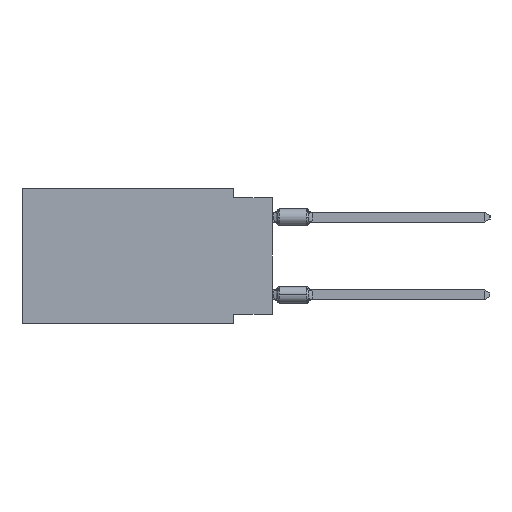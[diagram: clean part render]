
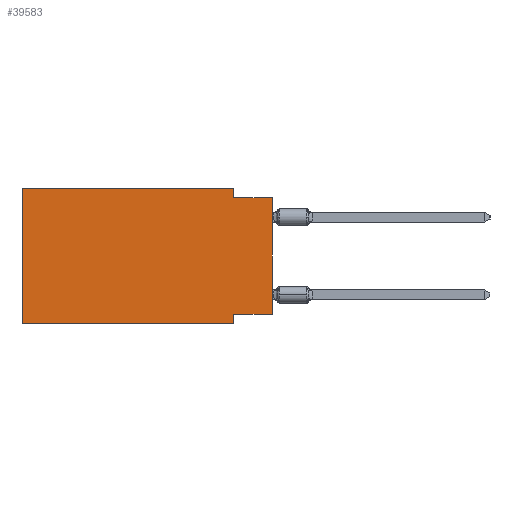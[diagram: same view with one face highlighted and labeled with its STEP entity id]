
A CAD part, left-side view. The second image highlights one B-rep face of the part: STEP entity #39583.
In plain terms, the highlighted planar face has unit normal (-1, 0, 0).
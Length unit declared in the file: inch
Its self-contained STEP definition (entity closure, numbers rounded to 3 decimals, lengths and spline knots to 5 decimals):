
#415 = CARTESIAN_POINT ( 'NONE',  ( 0., 0.1, -0.35 ) ) ;
#735 = DIRECTION ( 'NONE',  ( 0., 0., 1. ) ) ;
#1267 = FACE_OUTER_BOUND ( 'NONE', #35746, .T. ) ;
#1519 = VECTOR ( 'NONE', #735, 39.37008 ) ;
#1534 = EDGE_CURVE ( 'NONE', #35348, #14423, #10253, .T. ) ;
#1948 = EDGE_CURVE ( 'NONE', #33813, #29444, #14636, .T. ) ;
#2580 = DIRECTION ( 'NONE',  ( 0., -1., 0. ) ) ;
#2757 = CARTESIAN_POINT ( 'NONE',  ( 0., 0.1, -0.025 ) ) ;
#4021 = CARTESIAN_POINT ( 'NONE',  ( 0., 0., 0. ) ) ;
#4475 = LINE ( 'NONE', #37735, #1519 ) ;
#4509 = ORIENTED_EDGE ( 'NONE', *, *, #49030, .F. ) ;
#6438 = CARTESIAN_POINT ( 'NONE',  ( 0., 0.645, 0. ) ) ;
#8901 = VECTOR ( 'NONE', #40226, 39.37008 ) ;
#8943 = PLANE ( 'NONE',  #25062 ) ;
#10253 = LINE ( 'NONE', #26356, #43777 ) ;
#10476 = VERTEX_POINT ( 'NONE', #6438 ) ;
#10911 = ORIENTED_EDGE ( 'NONE', *, *, #32629, .F. ) ;
#11801 = DIRECTION ( 'NONE',  ( 0., 0., -1. ) ) ;
#12860 = CARTESIAN_POINT ( 'NONE',  ( 0., 0.1, -0.325 ) ) ;
#13354 = VECTOR ( 'NONE', #43729, 39.37008 ) ;
#13426 = LINE ( 'NONE', #28583, #13354 ) ;
#14423 = VERTEX_POINT ( 'NONE', #16208 ) ;
#14636 = LINE ( 'NONE', #48667, #8901 ) ;
#14691 = EDGE_CURVE ( 'NONE', #33813, #36939, #19634, .T. ) ;
#14749 = VERTEX_POINT ( 'NONE', #34278 ) ;
#16208 = CARTESIAN_POINT ( 'NONE',  ( 0., 0.1, -0.35 ) ) ;
#18506 = ORIENTED_EDGE ( 'NONE', *, *, #1534, .T. ) ;
#18625 = VECTOR ( 'NONE', #21934, 39.37008 ) ;
#19139 = DIRECTION ( 'NONE',  ( 0., 0., 1. ) ) ;
#19634 = LINE ( 'NONE', #4021, #46239 ) ;
#19869 = DIRECTION ( 'NONE',  ( 0., 0., -1. ) ) ;
#20236 = DIRECTION ( 'NONE',  ( 0., 0., -1. ) ) ;
#21934 = DIRECTION ( 'NONE',  ( 0., -1., 0. ) ) ;
#22164 = ORIENTED_EDGE ( 'NONE', *, *, #27296, .F. ) ;
#22923 = EDGE_CURVE ( 'NONE', #39631, #36939, #13426, .T. ) ;
#23052 = VECTOR ( 'NONE', #11801, 39.37008 ) ;
#23825 = DIRECTION ( 'NONE',  ( 1., 0., 0. ) ) ;
#23941 = LINE ( 'NONE', #39107, #30271 ) ;
#24239 = LINE ( 'NONE', #40804, #18625 ) ;
#25062 = AXIS2_PLACEMENT_3D ( 'NONE', #27317, #23825, #19869 ) ;
#26356 = CARTESIAN_POINT ( 'NONE',  ( 0., 0.645, -0.35 ) ) ;
#27194 = LINE ( 'NONE', #415, #23052 ) ;
#27296 = EDGE_CURVE ( 'NONE', #35348, #10476, #4475, .T. ) ;
#27317 = CARTESIAN_POINT ( 'NONE',  ( 0., 0.645, 0. ) ) ;
#28139 = ORIENTED_EDGE ( 'NONE', *, *, #42933, .F. ) ;
#28583 = CARTESIAN_POINT ( 'NONE',  ( 0., 0., -0.025 ) ) ;
#29444 = VERTEX_POINT ( 'NONE', #12860 ) ;
#29736 = CARTESIAN_POINT ( 'NONE',  ( 0., 0.645, -0.35 ) ) ;
#30271 = VECTOR ( 'NONE', #20236, 39.37008 ) ;
#32629 = EDGE_CURVE ( 'NONE', #14749, #39631, #23941, .T. ) ;
#33813 = VERTEX_POINT ( 'NONE', #45904 ) ;
#34278 = CARTESIAN_POINT ( 'NONE',  ( 0., 0.1, 0. ) ) ;
#34451 = ORIENTED_EDGE ( 'NONE', *, *, #22923, .F. ) ;
#34690 = CARTESIAN_POINT ( 'NONE',  ( 0., 0., -0.025 ) ) ;
#35348 = VERTEX_POINT ( 'NONE', #29736 ) ;
#35746 = EDGE_LOOP ( 'NONE', ( #46228, #34451, #10911, #4509, #22164, #18506, #28139, #48311 ) ) ;
#36939 = VERTEX_POINT ( 'NONE', #34690 ) ;
#37735 = CARTESIAN_POINT ( 'NONE',  ( 0., 0.645, 0. ) ) ;
#39107 = CARTESIAN_POINT ( 'NONE',  ( 0., 0.1, 0. ) ) ;
#39583 = ADVANCED_FACE ( 'NONE', ( #1267 ), #8943, .F. ) ;
#39631 = VERTEX_POINT ( 'NONE', #2757 ) ;
#40226 = DIRECTION ( 'NONE',  ( 0., 1., 0. ) ) ;
#40804 = CARTESIAN_POINT ( 'NONE',  ( 0., 0.645, 0. ) ) ;
#42933 = EDGE_CURVE ( 'NONE', #29444, #14423, #27194, .T. ) ;
#43729 = DIRECTION ( 'NONE',  ( 0., -1., 0. ) ) ;
#43777 = VECTOR ( 'NONE', #2580, 39.37008 ) ;
#45904 = CARTESIAN_POINT ( 'NONE',  ( 0., 0., -0.325 ) ) ;
#46228 = ORIENTED_EDGE ( 'NONE', *, *, #14691, .T. ) ;
#46239 = VECTOR ( 'NONE', #19139, 39.37008 ) ;
#48311 = ORIENTED_EDGE ( 'NONE', *, *, #1948, .F. ) ;
#48667 = CARTESIAN_POINT ( 'NONE',  ( 0., 0., -0.325 ) ) ;
#49030 = EDGE_CURVE ( 'NONE', #10476, #14749, #24239, .T. ) ;
